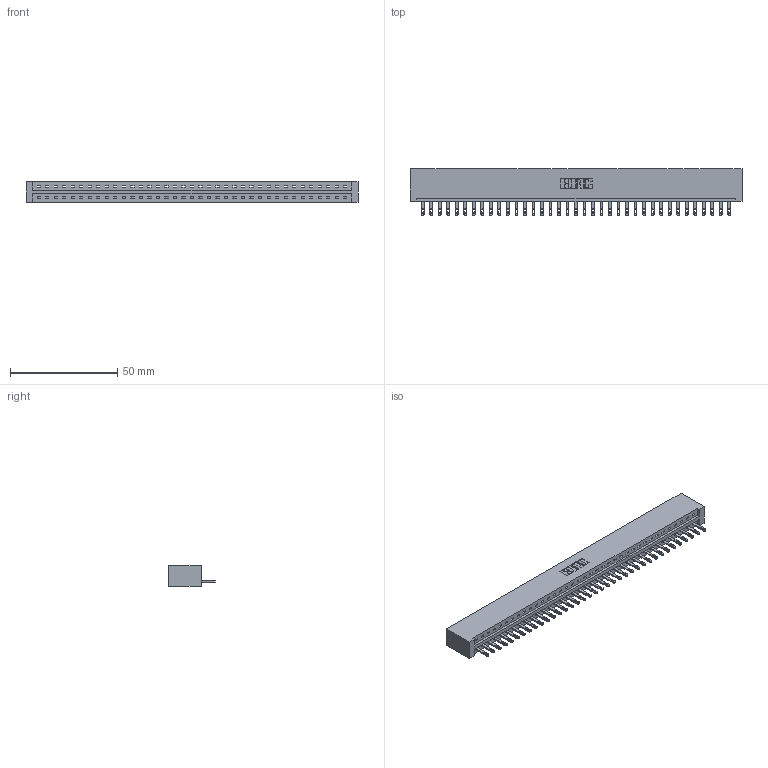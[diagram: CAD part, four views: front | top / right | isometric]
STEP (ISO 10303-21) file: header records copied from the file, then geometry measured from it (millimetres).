
FILE_DESCRIPTION (( 'STEP AP203' ), '1' );
FILE_NAME ('887-037-500-101.STEP', '2020-09-20T22:27:37', ( '' ), ( '' ), 'SwSTEP 2.0', 'SolidWorks 2020', '' );
FILE_SCHEMA (( 'CONFIG_CONTROL_DESIGN' ));
Length unit declared in the file: inch
Products named in the file (3): 837 Part_No Mounting Lugs; 887-037-500-101; 345-292-001_345-293-100
Assembly tree (38 placements, depth 2):
  887-037-500-101
    837 Part_No Mounting Lugs
    345-292-001_345-293-100  x37
Bounding box: 154.48 x 21.85 x 9.4 mm (x, y, z)
Volume: 16754.9 mm3; surface area: 17353.8 mm2
Topology: 38 solids, 38 shells, 2252 faces, 6947 edges, 4630 vertices
Faces by surface type: plane 1546, cylinder 706
Entity records: 27803 total; most frequent: CARTESIAN_POINT 4849, ORIENTED_EDGE 4822, DIRECTION 4085, EDGE_CURVE 2411, LINE 2287, VECTOR 2287, VERTEX_POINT 1606, AXIS2_PLACEMENT_3D 899
